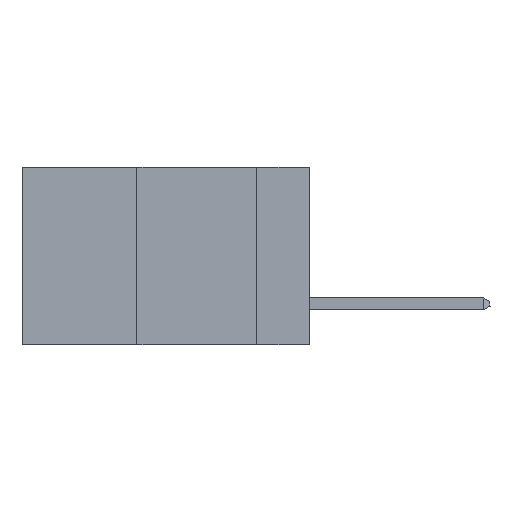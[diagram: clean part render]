
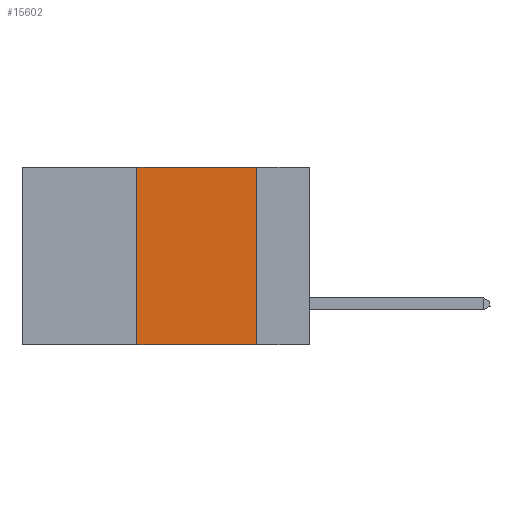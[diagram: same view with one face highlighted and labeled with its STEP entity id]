
A CAD part, left-side view. The second image highlights one B-rep face of the part: STEP entity #15602.
In plain terms, the highlighted planar face has unit normal (-1, 0, 0).
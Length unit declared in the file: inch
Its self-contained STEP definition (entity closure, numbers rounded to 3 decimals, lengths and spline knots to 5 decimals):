
#547 = ORIENTED_EDGE ( 'NONE', *, *, #37626, .F. ) ;
#5492 = LINE ( 'NONE', #14078, #30463 ) ;
#5902 = VECTOR ( 'NONE', #15748, 39.37008 ) ;
#8517 = VECTOR ( 'NONE', #40935, 39.37008 ) ;
#8728 = DIRECTION ( 'NONE',  ( 0., -1., 0. ) ) ;
#8931 = VERTEX_POINT ( 'NONE', #27401 ) ;
#11051 = AXIS2_PLACEMENT_3D ( 'NONE', #21603, #36084, #40463 ) ;
#12047 = CARTESIAN_POINT ( 'NONE',  ( 0., 0.11, -0.37 ) ) ;
#12213 = VECTOR ( 'NONE', #8728, 39.37008 ) ;
#12346 = EDGE_CURVE ( 'NONE', #40239, #30120, #18833, .T. ) ;
#14078 = CARTESIAN_POINT ( 'NONE',  ( 0., 0.6, 0. ) ) ;
#15602 = ADVANCED_FACE ( 'NONE', ( #42865 ), #35097, .F. ) ;
#15748 = DIRECTION ( 'NONE',  ( 0., 0., 1. ) ) ;
#15828 = VERTEX_POINT ( 'NONE', #28995 ) ;
#15870 = ORIENTED_EDGE ( 'NONE', *, *, #25117, .F. ) ;
#17908 = LINE ( 'NONE', #45098, #8517 ) ;
#18541 = LINE ( 'NONE', #22736, #5902 ) ;
#18833 = LINE ( 'NONE', #22993, #12213 ) ;
#21603 = CARTESIAN_POINT ( 'NONE',  ( 0., 0.6, 0. ) ) ;
#22736 = CARTESIAN_POINT ( 'NONE',  ( 0., 0.36, 0. ) ) ;
#22993 = CARTESIAN_POINT ( 'NONE',  ( 0., 0.6, -0.37 ) ) ;
#25117 = EDGE_CURVE ( 'NONE', #15828, #30120, #17908, .T. ) ;
#27401 = CARTESIAN_POINT ( 'NONE',  ( 0., 0.36, 0. ) ) ;
#27446 = EDGE_LOOP ( 'NONE', ( #15870, #43217, #547, #30971 ) ) ;
#28995 = CARTESIAN_POINT ( 'NONE',  ( 0., 0.11, 0. ) ) ;
#30063 = CARTESIAN_POINT ( 'NONE',  ( 0., 0.36, -0.37 ) ) ;
#30120 = VERTEX_POINT ( 'NONE', #12047 ) ;
#30463 = VECTOR ( 'NONE', #37563, 39.37008 ) ;
#30971 = ORIENTED_EDGE ( 'NONE', *, *, #12346, .T. ) ;
#32879 = EDGE_CURVE ( 'NONE', #8931, #15828, #5492, .T. ) ;
#35097 = PLANE ( 'NONE',  #11051 ) ;
#36084 = DIRECTION ( 'NONE',  ( 1., 0., 0. ) ) ;
#37563 = DIRECTION ( 'NONE',  ( 0., -1., 0. ) ) ;
#37626 = EDGE_CURVE ( 'NONE', #40239, #8931, #18541, .T. ) ;
#40239 = VERTEX_POINT ( 'NONE', #30063 ) ;
#40463 = DIRECTION ( 'NONE',  ( 0., 0., -1. ) ) ;
#40935 = DIRECTION ( 'NONE',  ( 0., 0., -1. ) ) ;
#42865 = FACE_OUTER_BOUND ( 'NONE', #27446, .T. ) ;
#43217 = ORIENTED_EDGE ( 'NONE', *, *, #32879, .F. ) ;
#45098 = CARTESIAN_POINT ( 'NONE',  ( 0., 0.11, 0. ) ) ;
